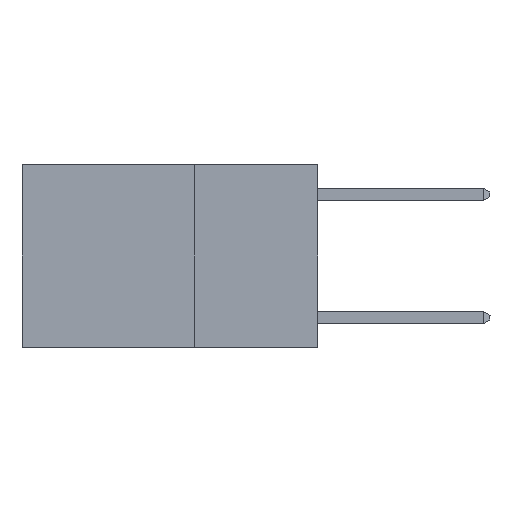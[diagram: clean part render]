
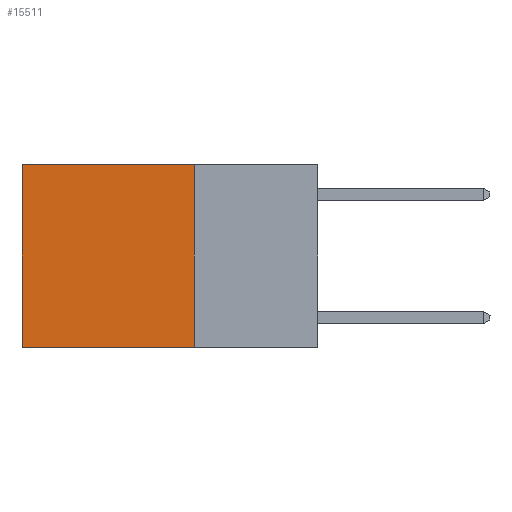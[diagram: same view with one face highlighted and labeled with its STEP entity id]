
A CAD part, left-side view. The second image highlights one B-rep face of the part: STEP entity #15511.
In plain terms, the highlighted planar face has unit normal (-1, 0, 0).
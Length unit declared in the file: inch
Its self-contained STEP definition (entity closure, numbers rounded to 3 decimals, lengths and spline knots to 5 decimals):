
#709 = VERTEX_POINT ( 'NONE', #12630 ) ;
#823 = DIRECTION ( 'NONE',  ( 0., 0., -1. ) ) ;
#1302 = DIRECTION ( 'NONE',  ( 0., 0., -1. ) ) ;
#1387 = CARTESIAN_POINT ( 'NONE',  ( 0.2625, 0.6, 0. ) ) ;
#1660 = VECTOR ( 'NONE', #14541, 39.37008 ) ;
#2308 = LINE ( 'NONE', #18570, #1660 ) ;
#3847 = VERTEX_POINT ( 'NONE', #6418 ) ;
#3854 = ORIENTED_EDGE ( 'NONE', *, *, #22860, .T. ) ;
#3866 = LINE ( 'NONE', #5675, #13951 ) ;
#4524 = ORIENTED_EDGE ( 'NONE', *, *, #17244, .F. ) ;
#4779 = VERTEX_POINT ( 'NONE', #16608 ) ;
#4826 = ORIENTED_EDGE ( 'NONE', *, *, #23925, .F. ) ;
#5675 = CARTESIAN_POINT ( 'NONE',  ( 0.2625, 0.25, -0.37 ) ) ;
#6310 = VECTOR ( 'NONE', #1302, 39.37008 ) ;
#6418 = CARTESIAN_POINT ( 'NONE',  ( 0.2625, 0.25, -0.37 ) ) ;
#6778 = ORIENTED_EDGE ( 'NONE', *, *, #12719, .T. ) ;
#7734 = DIRECTION ( 'NONE',  ( 0., 1., 0. ) ) ;
#10451 = CARTESIAN_POINT ( 'NONE',  ( 0.2625, 0.25, 0. ) ) ;
#12630 = CARTESIAN_POINT ( 'NONE',  ( 0.2625, 0.6, 0. ) ) ;
#12719 = EDGE_CURVE ( 'NONE', #4779, #709, #23756, .T. ) ;
#13001 = DIRECTION ( 'NONE',  ( 1., 0., 0. ) ) ;
#13242 = VECTOR ( 'NONE', #14399, 39.37008 ) ;
#13871 = VERTEX_POINT ( 'NONE', #17764 ) ;
#13951 = VECTOR ( 'NONE', #7734, 39.37008 ) ;
#14399 = DIRECTION ( 'NONE',  ( 0., 1., 0. ) ) ;
#14541 = DIRECTION ( 'NONE',  ( 0., 0., -1. ) ) ;
#15511 = ADVANCED_FACE ( 'NONE', ( #16195 ), #24786, .F. ) ;
#16195 = FACE_OUTER_BOUND ( 'NONE', #22616, .T. ) ;
#16608 = CARTESIAN_POINT ( 'NONE',  ( 0.2625, 0.25, 0. ) ) ;
#17244 = EDGE_CURVE ( 'NONE', #3847, #13871, #3866, .T. ) ;
#17764 = CARTESIAN_POINT ( 'NONE',  ( 0.2625, 0.6, -0.37 ) ) ;
#18570 = CARTESIAN_POINT ( 'NONE',  ( 0.2625, 0.25, 0. ) ) ;
#18859 = LINE ( 'NONE', #1387, #6310 ) ;
#20895 = CARTESIAN_POINT ( 'NONE',  ( 0.2625, 0.25, 0. ) ) ;
#22237 = AXIS2_PLACEMENT_3D ( 'NONE', #20895, #13001, #823 ) ;
#22616 = EDGE_LOOP ( 'NONE', ( #3854, #4524, #4826, #6778 ) ) ;
#22860 = EDGE_CURVE ( 'NONE', #709, #13871, #18859, .T. ) ;
#23756 = LINE ( 'NONE', #10451, #13242 ) ;
#23925 = EDGE_CURVE ( 'NONE', #4779, #3847, #2308, .T. ) ;
#24786 = PLANE ( 'NONE',  #22237 ) ;
